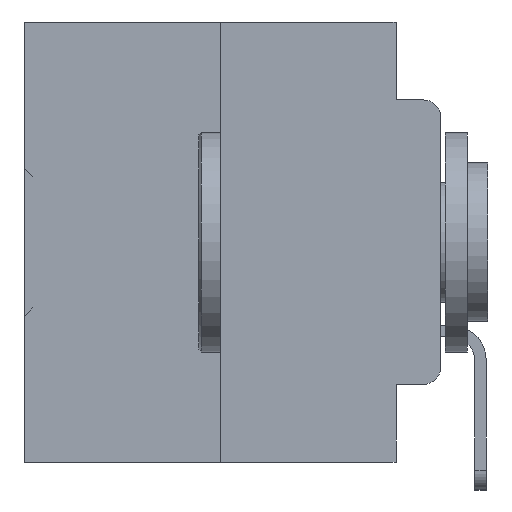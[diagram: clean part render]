
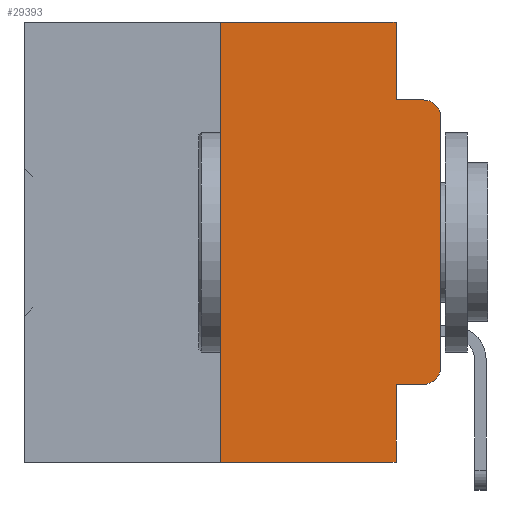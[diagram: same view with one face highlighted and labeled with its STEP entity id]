
A CAD part, left-side view. The second image highlights one B-rep face of the part: STEP entity #29393.
In plain terms, the highlighted planar face has unit normal (-1, 0, 0).
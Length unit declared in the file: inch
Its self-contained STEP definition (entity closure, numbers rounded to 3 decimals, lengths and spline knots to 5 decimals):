
#331 = CARTESIAN_POINT ( 'NONE',  ( 0., 0.051, -0.5 ) ) ;
#423 = VERTEX_POINT ( 'NONE', #18936 ) ;
#469 = EDGE_LOOP ( 'NONE', ( #34754, #4806, #36535, #10417, #25809, #5310, #28507, #33893, #3897, #6727 ) ) ;
#528 = CARTESIAN_POINT ( 'NONE',  ( 0., 0.051, -0.4115 ) ) ;
#986 = CARTESIAN_POINT ( 'NONE',  ( 0., 0.051, 0. ) ) ;
#1669 = AXIS2_PLACEMENT_3D ( 'NONE', #8226, #28481, #11188 ) ;
#2008 = VERTEX_POINT ( 'NONE', #6270 ) ;
#2645 = CARTESIAN_POINT ( 'NONE',  ( 0., 0.25, 0. ) ) ;
#3070 = VERTEX_POINT ( 'NONE', #2645 ) ;
#3686 = CARTESIAN_POINT ( 'NONE',  ( 0., 0., 0. ) ) ;
#3897 = ORIENTED_EDGE ( 'NONE', *, *, #19362, .T. ) ;
#4640 = VERTEX_POINT ( 'NONE', #6054 ) ;
#4641 = LINE ( 'NONE', #32357, #34614 ) ;
#4806 = ORIENTED_EDGE ( 'NONE', *, *, #12759, .T. ) ;
#5030 = CARTESIAN_POINT ( 'NONE',  ( 0., 0.051, -0.4115 ) ) ;
#5310 = ORIENTED_EDGE ( 'NONE', *, *, #29933, .F. ) ;
#6054 = CARTESIAN_POINT ( 'NONE',  ( 0., 0.02, -0.0885 ) ) ;
#6270 = CARTESIAN_POINT ( 'NONE',  ( 0., 0.051, 0. ) ) ;
#6727 = ORIENTED_EDGE ( 'NONE', *, *, #16353, .T. ) ;
#6960 = VECTOR ( 'NONE', #18139, 39.37008 ) ;
#7786 = CARTESIAN_POINT ( 'NONE',  ( 0., 0., -0.3915 ) ) ;
#8226 = CARTESIAN_POINT ( 'NONE',  ( 0., 0.02, -0.3915 ) ) ;
#8336 = EDGE_CURVE ( 'NONE', #423, #4640, #35646, .T. ) ;
#9283 = CARTESIAN_POINT ( 'NONE',  ( 0., 0.051, 0. ) ) ;
#10417 = ORIENTED_EDGE ( 'NONE', *, *, #22942, .F. ) ;
#11098 = VECTOR ( 'NONE', #18356, 39.37008 ) ;
#11188 = DIRECTION ( 'NONE',  ( 0., 0., -1. ) ) ;
#11522 = CARTESIAN_POINT ( 'NONE',  ( 0., 0.02, -0.1085 ) ) ;
#11808 = CIRCLE ( 'NONE', #1669, 0.02 ) ;
#12019 = LINE ( 'NONE', #3686, #11098 ) ;
#12136 = DIRECTION ( 'NONE',  ( 1., 0., 0. ) ) ;
#12146 = VECTOR ( 'NONE', #23917, 39.37008 ) ;
#12235 = DIRECTION ( 'NONE',  ( 0., 0., 1. ) ) ;
#12256 = DIRECTION ( 'NONE',  ( 0., 0., -1. ) ) ;
#12759 = EDGE_CURVE ( 'NONE', #13688, #4640, #19721, .T. ) ;
#12944 = VERTEX_POINT ( 'NONE', #331 ) ;
#12998 = DIRECTION ( 'NONE',  ( 0., 0., -1. ) ) ;
#13515 = DIRECTION ( 'NONE',  ( 0., -1., 0. ) ) ;
#13688 = VERTEX_POINT ( 'NONE', #17721 ) ;
#14360 = EDGE_CURVE ( 'NONE', #3070, #2008, #15514, .T. ) ;
#14391 = DIRECTION ( 'NONE',  ( 0., 0., -1. ) ) ;
#15514 = LINE ( 'NONE', #23472, #20498 ) ;
#15860 = VERTEX_POINT ( 'NONE', #37623 ) ;
#16353 = EDGE_CURVE ( 'NONE', #23531, #29106, #11808, .T. ) ;
#17721 = CARTESIAN_POINT ( 'NONE',  ( 0., 0., -0.1085 ) ) ;
#18139 = DIRECTION ( 'NONE',  ( 0., -1., 0. ) ) ;
#18154 = EDGE_CURVE ( 'NONE', #19552, #12944, #27498, .T. ) ;
#18356 = DIRECTION ( 'NONE',  ( 0., 0., 1. ) ) ;
#18936 = CARTESIAN_POINT ( 'NONE',  ( 0., 0.051, -0.0885 ) ) ;
#19362 = EDGE_CURVE ( 'NONE', #19552, #23531, #22454, .T. ) ;
#19552 = VERTEX_POINT ( 'NONE', #5030 ) ;
#19721 = CIRCLE ( 'NONE', #20352, 0.02 ) ;
#19763 = CARTESIAN_POINT ( 'NONE',  ( 0., 0.02, -0.4115 ) ) ;
#19912 = EDGE_CURVE ( 'NONE', #29106, #13688, #12019, .T. ) ;
#20352 = AXIS2_PLACEMENT_3D ( 'NONE', #11522, #31619, #14391 ) ;
#20498 = VECTOR ( 'NONE', #26372, 39.37008 ) ;
#20742 = LINE ( 'NONE', #21021, #12146 ) ;
#20929 = VECTOR ( 'NONE', #12998, 39.37008 ) ;
#21021 = CARTESIAN_POINT ( 'NONE',  ( 0., 0.473, -0.5 ) ) ;
#22454 = LINE ( 'NONE', #528, #6960 ) ;
#22942 = EDGE_CURVE ( 'NONE', #2008, #423, #29468, .T. ) ;
#23472 = CARTESIAN_POINT ( 'NONE',  ( 0., 0.473, 0. ) ) ;
#23531 = VERTEX_POINT ( 'NONE', #19763 ) ;
#23642 = PLANE ( 'NONE',  #27724 ) ;
#23917 = DIRECTION ( 'NONE',  ( 0., -1., 0. ) ) ;
#25028 = CARTESIAN_POINT ( 'NONE',  ( 0., 0.051, -0.0885 ) ) ;
#25809 = ORIENTED_EDGE ( 'NONE', *, *, #14360, .F. ) ;
#26372 = DIRECTION ( 'NONE',  ( 0., -1., 0. ) ) ;
#26601 = VECTOR ( 'NONE', #12256, 39.37008 ) ;
#27081 = EDGE_CURVE ( 'NONE', #15860, #12944, #20742, .T. ) ;
#27498 = LINE ( 'NONE', #9283, #26601 ) ;
#27724 = AXIS2_PLACEMENT_3D ( 'NONE', #29388, #12136, #32265 ) ;
#28481 = DIRECTION ( 'NONE',  ( -1., 0., 0. ) ) ;
#28507 = ORIENTED_EDGE ( 'NONE', *, *, #27081, .T. ) ;
#29106 = VERTEX_POINT ( 'NONE', #7786 ) ;
#29388 = CARTESIAN_POINT ( 'NONE',  ( 0., 0.473, 0. ) ) ;
#29393 = ADVANCED_FACE ( 'NONE', ( #31475 ), #23642, .F. ) ;
#29468 = LINE ( 'NONE', #986, #20929 ) ;
#29933 = EDGE_CURVE ( 'NONE', #15860, #3070, #4641, .T. ) ;
#31475 = FACE_OUTER_BOUND ( 'NONE', #469, .T. ) ;
#31619 = DIRECTION ( 'NONE',  ( -1., 0., 0. ) ) ;
#32265 = DIRECTION ( 'NONE',  ( 0., 0., -1. ) ) ;
#32357 = CARTESIAN_POINT ( 'NONE',  ( 0., 0.25, 0. ) ) ;
#32957 = VECTOR ( 'NONE', #13515, 39.37008 ) ;
#33893 = ORIENTED_EDGE ( 'NONE', *, *, #18154, .F. ) ;
#34614 = VECTOR ( 'NONE', #12235, 39.37008 ) ;
#34754 = ORIENTED_EDGE ( 'NONE', *, *, #19912, .T. ) ;
#35646 = LINE ( 'NONE', #25028, #32957 ) ;
#36535 = ORIENTED_EDGE ( 'NONE', *, *, #8336, .F. ) ;
#37623 = CARTESIAN_POINT ( 'NONE',  ( 0., 0.25, -0.5 ) ) ;
